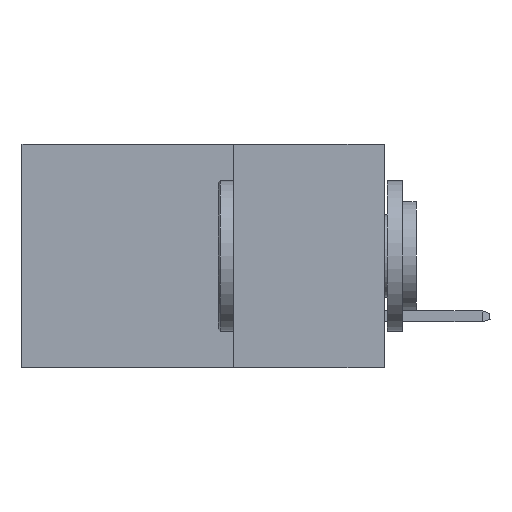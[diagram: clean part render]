
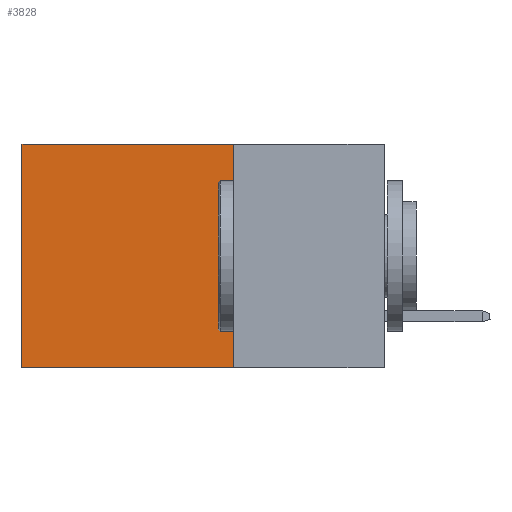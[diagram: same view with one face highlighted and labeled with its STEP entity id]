
A CAD part, left-side view. The second image highlights one B-rep face of the part: STEP entity #3828.
In plain terms, the highlighted planar face has unit normal (-1, 0, 0).
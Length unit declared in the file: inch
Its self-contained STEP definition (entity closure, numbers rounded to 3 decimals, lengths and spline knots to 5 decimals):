
#26 = DIRECTION ( 'NONE',  ( 0., 0., -1. ) ) ;
#135 = CARTESIAN_POINT ( 'NONE',  ( 0.298, 0.25, 0. ) ) ;
#621 = DIRECTION ( 'NONE',  ( 0., 1., 0. ) ) ;
#811 = DIRECTION ( 'NONE',  ( 0., 0., -1. ) ) ;
#1398 = AXIS2_PLACEMENT_3D ( 'NONE', #6179, #5263, #26 ) ;
#2003 = EDGE_LOOP ( 'NONE', ( #8590, #6865, #4412, #2361 ) ) ;
#2361 = ORIENTED_EDGE ( 'NONE', *, *, #2678, .T. ) ;
#2678 = EDGE_CURVE ( 'NONE', #3254, #8262, #8153, .T. ) ;
#3254 = VERTEX_POINT ( 'NONE', #4512 ) ;
#3387 = LINE ( 'NONE', #8564, #7282 ) ;
#3558 = VECTOR ( 'NONE', #621, 39.37008 ) ;
#3828 = ADVANCED_FACE ( 'NONE', ( #7806 ), #4600, .F. ) ;
#4120 = CARTESIAN_POINT ( 'NONE',  ( 0.298, 0.25, -0.37 ) ) ;
#4412 = ORIENTED_EDGE ( 'NONE', *, *, #8662, .F. ) ;
#4490 = LINE ( 'NONE', #5808, #8651 ) ;
#4512 = CARTESIAN_POINT ( 'NONE',  ( 0.298, 0.25, 0. ) ) ;
#4600 = PLANE ( 'NONE',  #1398 ) ;
#4848 = CARTESIAN_POINT ( 'NONE',  ( 0.298, 0.6, -0.37 ) ) ;
#5263 = DIRECTION ( 'NONE',  ( 1., 0., 0. ) ) ;
#5808 = CARTESIAN_POINT ( 'NONE',  ( 0.298, 0.25, -0.37 ) ) ;
#6179 = CARTESIAN_POINT ( 'NONE',  ( 0.298, 0.25, 0. ) ) ;
#6181 = EDGE_CURVE ( 'NONE', #8262, #6267, #3387, .T. ) ;
#6267 = VERTEX_POINT ( 'NONE', #4848 ) ;
#6746 = VECTOR ( 'NONE', #811, 39.37008 ) ;
#6865 = ORIENTED_EDGE ( 'NONE', *, *, #8032, .F. ) ;
#7237 = VERTEX_POINT ( 'NONE', #4120 ) ;
#7282 = VECTOR ( 'NONE', #7768, 39.37008 ) ;
#7768 = DIRECTION ( 'NONE',  ( 0., 0., -1. ) ) ;
#7806 = FACE_OUTER_BOUND ( 'NONE', #2003, .T. ) ;
#8032 = EDGE_CURVE ( 'NONE', #7237, #6267, #4490, .T. ) ;
#8153 = LINE ( 'NONE', #9746, #3558 ) ;
#8185 = CARTESIAN_POINT ( 'NONE',  ( 0.298, 0.6, 0. ) ) ;
#8262 = VERTEX_POINT ( 'NONE', #8185 ) ;
#8564 = CARTESIAN_POINT ( 'NONE',  ( 0.298, 0.6, 0. ) ) ;
#8590 = ORIENTED_EDGE ( 'NONE', *, *, #6181, .T. ) ;
#8651 = VECTOR ( 'NONE', #9521, 39.37008 ) ;
#8662 = EDGE_CURVE ( 'NONE', #3254, #7237, #9261, .T. ) ;
#9261 = LINE ( 'NONE', #135, #6746 ) ;
#9521 = DIRECTION ( 'NONE',  ( 0., 1., 0. ) ) ;
#9746 = CARTESIAN_POINT ( 'NONE',  ( 0.298, 0.25, 0. ) ) ;
